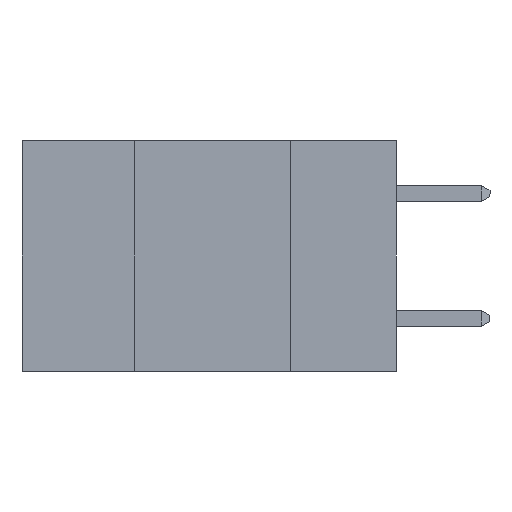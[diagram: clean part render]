
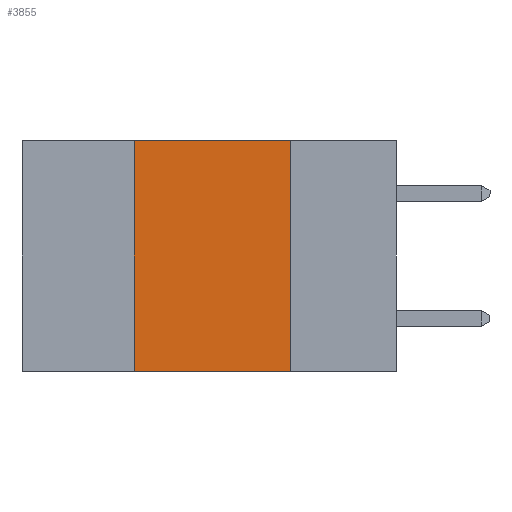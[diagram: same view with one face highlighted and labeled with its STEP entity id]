
A CAD part, left-side view. The second image highlights one B-rep face of the part: STEP entity #3855.
In plain terms, the highlighted planar face has unit normal (-1, 0, 0).
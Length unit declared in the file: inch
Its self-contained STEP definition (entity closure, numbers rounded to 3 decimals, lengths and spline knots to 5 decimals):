
#322 = VERTEX_POINT ( 'NONE', #2420 ) ;
#556 = ORIENTED_EDGE ( 'NONE', *, *, #2676, .F. ) ;
#1001 = EDGE_CURVE ( 'NONE', #3539, #6878, #4485, .T. ) ;
#1041 = DIRECTION ( 'NONE',  ( 0., 0., -1. ) ) ;
#1177 = CARTESIAN_POINT ( 'NONE',  ( 0., 0.6, 0. ) ) ;
#1182 = LINE ( 'NONE', #1747, #3895 ) ;
#1283 = CARTESIAN_POINT ( 'NONE',  ( 0., 0.17, 0. ) ) ;
#1564 = DIRECTION ( 'NONE',  ( 0., 0., -1. ) ) ;
#1674 = EDGE_LOOP ( 'NONE', ( #556, #3205, #4367, #4185 ) ) ;
#1747 = CARTESIAN_POINT ( 'NONE',  ( 0., 0.17, -0.37 ) ) ;
#2222 = LINE ( 'NONE', #2845, #8620 ) ;
#2420 = CARTESIAN_POINT ( 'NONE',  ( 0., 0.42, -0.37 ) ) ;
#2676 = EDGE_CURVE ( 'NONE', #6878, #5992, #1182, .T. ) ;
#2845 = CARTESIAN_POINT ( 'NONE',  ( 0., 0.6, -0.37 ) ) ;
#3090 = LINE ( 'NONE', #3693, #5625 ) ;
#3099 = AXIS2_PLACEMENT_3D ( 'NONE', #7475, #6877, #1564 ) ;
#3205 = ORIENTED_EDGE ( 'NONE', *, *, #1001, .F. ) ;
#3539 = VERTEX_POINT ( 'NONE', #6514 ) ;
#3693 = CARTESIAN_POINT ( 'NONE',  ( 0., 0.42, -0.37 ) ) ;
#3855 = ADVANCED_FACE ( 'NONE', ( #7325 ), #6153, .F. ) ;
#3895 = VECTOR ( 'NONE', #1041, 39.37008 ) ;
#4185 = ORIENTED_EDGE ( 'NONE', *, *, #7277, .T. ) ;
#4367 = ORIENTED_EDGE ( 'NONE', *, *, #7869, .F. ) ;
#4485 = LINE ( 'NONE', #1177, #7532 ) ;
#4777 = DIRECTION ( 'NONE',  ( 0., -1., 0. ) ) ;
#5625 = VECTOR ( 'NONE', #7800, 39.37008 ) ;
#5992 = VERTEX_POINT ( 'NONE', #7145 ) ;
#6153 = PLANE ( 'NONE',  #3099 ) ;
#6514 = CARTESIAN_POINT ( 'NONE',  ( 0., 0.42, 0. ) ) ;
#6877 = DIRECTION ( 'NONE',  ( 1., 0., 0. ) ) ;
#6878 = VERTEX_POINT ( 'NONE', #1283 ) ;
#7145 = CARTESIAN_POINT ( 'NONE',  ( 0., 0.17, -0.37 ) ) ;
#7277 = EDGE_CURVE ( 'NONE', #322, #5992, #2222, .T. ) ;
#7325 = FACE_OUTER_BOUND ( 'NONE', #1674, .T. ) ;
#7475 = CARTESIAN_POINT ( 'NONE',  ( 0., 0.6, 0. ) ) ;
#7532 = VECTOR ( 'NONE', #7861, 39.37008 ) ;
#7800 = DIRECTION ( 'NONE',  ( 0., 0., 1. ) ) ;
#7861 = DIRECTION ( 'NONE',  ( 0., -1., 0. ) ) ;
#7869 = EDGE_CURVE ( 'NONE', #322, #3539, #3090, .T. ) ;
#8620 = VECTOR ( 'NONE', #4777, 39.37008 ) ;
